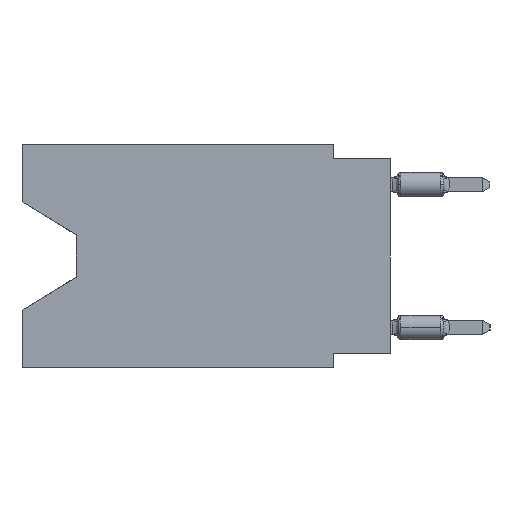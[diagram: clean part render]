
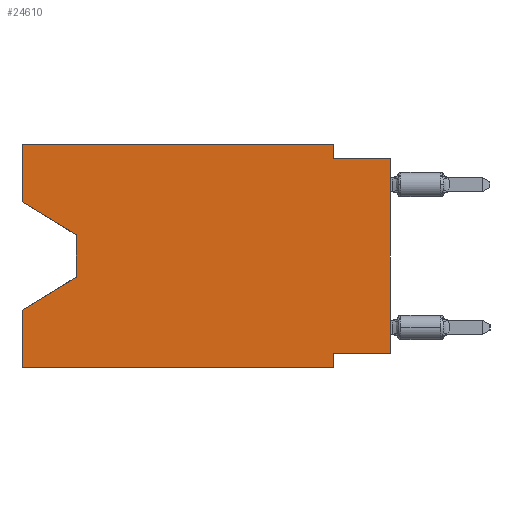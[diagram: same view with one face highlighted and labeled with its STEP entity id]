
A CAD part, left-side view. The second image highlights one B-rep face of the part: STEP entity #24610.
In plain terms, the highlighted planar face has unit normal (-1, 0, 0).
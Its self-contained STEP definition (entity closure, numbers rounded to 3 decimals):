
#326 = CARTESIAN_POINT ( 'NONE',  ( 0., 0., 0. ) ) ;
#1478 = CARTESIAN_POINT ( 'NONE',  ( 0., 16.383, -9.906 ) ) ;
#2300 = EDGE_CURVE ( 'NONE', #13877, #27841, #21555, .T. ) ;
#2341 = ORIENTED_EDGE ( 'NONE', *, *, #12382, .T. ) ;
#2949 = DIRECTION ( 'NONE',  ( 0., -1., 0. ) ) ;
#4019 = CARTESIAN_POINT ( 'NONE',  ( 0., 16.383, 0. ) ) ;
#5194 = VECTOR ( 'NONE', #12297, 1000. ) ;
#5306 = LINE ( 'NONE', #8620, #13654 ) ;
#5912 = VERTEX_POINT ( 'NONE', #15106 ) ;
#6220 = VECTOR ( 'NONE', #15846, 1000. ) ;
#6230 = EDGE_CURVE ( 'NONE', #9667, #5912, #23600, .T. ) ;
#7254 = AXIS2_PLACEMENT_3D ( 'NONE', #31137, #18847, #9213 ) ;
#7449 = CARTESIAN_POINT ( 'NONE',  ( 0., 0., -0.635 ) ) ;
#7759 = DIRECTION ( 'NONE',  ( 0., 0., 1. ) ) ;
#7861 = CARTESIAN_POINT ( 'NONE',  ( 0., 2.54, -9.271 ) ) ;
#7960 = VERTEX_POINT ( 'NONE', #19736 ) ;
#8156 = DIRECTION ( 'NONE',  ( 0., 0., 1. ) ) ;
#8190 = LINE ( 'NONE', #27439, #19016 ) ;
#8208 = ORIENTED_EDGE ( 'NONE', *, *, #6230, .F. ) ;
#8586 = VECTOR ( 'NONE', #8156, 1000. ) ;
#8620 = CARTESIAN_POINT ( 'NONE',  ( 0., 13.97, -5.893 ) ) ;
#8737 = CARTESIAN_POINT ( 'NONE',  ( 0., 16.383, -2.546 ) ) ;
#9008 = VECTOR ( 'NONE', #30853, 1000. ) ;
#9213 = DIRECTION ( 'NONE',  ( 0., 0., -1. ) ) ;
#9254 = DIRECTION ( 'NONE',  ( 0., 0., -1. ) ) ;
#9667 = VERTEX_POINT ( 'NONE', #7861 ) ;
#9680 = PLANE ( 'NONE',  #7254 ) ;
#10047 = LINE ( 'NONE', #1478, #26057 ) ;
#10245 = VECTOR ( 'NONE', #9254, 1000. ) ;
#10499 = DIRECTION ( 'NONE',  ( 0., 0.855, -0.519 ) ) ;
#11069 = VERTEX_POINT ( 'NONE', #30880 ) ;
#11603 = CARTESIAN_POINT ( 'NONE',  ( 0., 2.54, -9.906 ) ) ;
#12297 = DIRECTION ( 'NONE',  ( 0., -0.855, -0.519 ) ) ;
#12382 = EDGE_CURVE ( 'NONE', #27841, #31205, #5306, .T. ) ;
#12437 = ORIENTED_EDGE ( 'NONE', *, *, #2300, .T. ) ;
#12693 = CARTESIAN_POINT ( 'NONE',  ( 0., 13.97, -4.013 ) ) ;
#13144 = EDGE_CURVE ( 'NONE', #11069, #30994, #14709, .T. ) ;
#13451 = CARTESIAN_POINT ( 'NONE',  ( 0., 16.383, -7.36 ) ) ;
#13635 = ORIENTED_EDGE ( 'NONE', *, *, #25833, .F. ) ;
#13641 = EDGE_CURVE ( 'NONE', #26118, #16087, #27875, .T. ) ;
#13654 = VECTOR ( 'NONE', #10499, 1000. ) ;
#13877 = VERTEX_POINT ( 'NONE', #12693 ) ;
#14334 = VECTOR ( 'NONE', #23282, 1000. ) ;
#14366 = LINE ( 'NONE', #28882, #5194 ) ;
#14709 = LINE ( 'NONE', #326, #20678 ) ;
#15106 = CARTESIAN_POINT ( 'NONE',  ( 0., 2.54, -9.906 ) ) ;
#15130 = EDGE_CURVE ( 'NONE', #31153, #5912, #10047, .T. ) ;
#15409 = CARTESIAN_POINT ( 'NONE',  ( 0., 16.383, 0. ) ) ;
#15824 = CARTESIAN_POINT ( 'NONE',  ( 0., 16.383, -9.906 ) ) ;
#15846 = DIRECTION ( 'NONE',  ( 0., 0., 1. ) ) ;
#16087 = VERTEX_POINT ( 'NONE', #30303 ) ;
#17230 = LINE ( 'NONE', #7449, #30895 ) ;
#18193 = CARTESIAN_POINT ( 'NONE',  ( 0., 13.97, -5.893 ) ) ;
#18832 = LINE ( 'NONE', #28458, #6220 ) ;
#18847 = DIRECTION ( 'NONE',  ( 1., 0., 0. ) ) ;
#19016 = VECTOR ( 'NONE', #25064, 1000. ) ;
#19604 = ORIENTED_EDGE ( 'NONE', *, *, #15130, .T. ) ;
#19736 = CARTESIAN_POINT ( 'NONE',  ( 0., 2.54, -0.635 ) ) ;
#20631 = CARTESIAN_POINT ( 'NONE',  ( 0., 2.54, 0. ) ) ;
#20678 = VECTOR ( 'NONE', #7759, 1000. ) ;
#20753 = EDGE_CURVE ( 'NONE', #31153, #31205, #18832, .T. ) ;
#20844 = EDGE_CURVE ( 'NONE', #7960, #30994, #17230, .T. ) ;
#21297 = EDGE_CURVE ( 'NONE', #26118, #13877, #14366, .T. ) ;
#21345 = ORIENTED_EDGE ( 'NONE', *, *, #13144, .T. ) ;
#21555 = LINE ( 'NONE', #28512, #10245 ) ;
#21976 = CARTESIAN_POINT ( 'NONE',  ( 0., 0., -0.635 ) ) ;
#22077 = ORIENTED_EDGE ( 'NONE', *, *, #20844, .F. ) ;
#23282 = DIRECTION ( 'NONE',  ( 0., -1., 0. ) ) ;
#23460 = ORIENTED_EDGE ( 'NONE', *, *, #20753, .F. ) ;
#23600 = LINE ( 'NONE', #11603, #9008 ) ;
#23917 = ORIENTED_EDGE ( 'NONE', *, *, #29962, .F. ) ;
#24467 = EDGE_CURVE ( 'NONE', #16087, #27168, #25177, .T. ) ;
#24502 = DIRECTION ( 'NONE',  ( 0., -1., 0. ) ) ;
#24573 = ORIENTED_EDGE ( 'NONE', *, *, #24467, .F. ) ;
#24610 = ADVANCED_FACE ( 'NONE', ( #28326 ), #9680, .F. ) ;
#25046 = EDGE_LOOP ( 'NONE', ( #25277, #12437, #2341, #23460, #19604, #8208, #13635, #21345, #22077, #23917, #24573, #27408 ) ) ;
#25064 = DIRECTION ( 'NONE',  ( 0., 0., -1. ) ) ;
#25177 = LINE ( 'NONE', #4019, #14334 ) ;
#25277 = ORIENTED_EDGE ( 'NONE', *, *, #21297, .T. ) ;
#25833 = EDGE_CURVE ( 'NONE', #11069, #9667, #26417, .T. ) ;
#26057 = VECTOR ( 'NONE', #2949, 1000. ) ;
#26118 = VERTEX_POINT ( 'NONE', #8737 ) ;
#26417 = LINE ( 'NONE', #26563, #29997 ) ;
#26563 = CARTESIAN_POINT ( 'NONE',  ( 0., 0., -9.271 ) ) ;
#27168 = VERTEX_POINT ( 'NONE', #20631 ) ;
#27408 = ORIENTED_EDGE ( 'NONE', *, *, #13641, .F. ) ;
#27439 = CARTESIAN_POINT ( 'NONE',  ( 0., 2.54, 0. ) ) ;
#27841 = VERTEX_POINT ( 'NONE', #18193 ) ;
#27875 = LINE ( 'NONE', #15409, #8586 ) ;
#28326 = FACE_OUTER_BOUND ( 'NONE', #25046, .T. ) ;
#28458 = CARTESIAN_POINT ( 'NONE',  ( 0., 16.383, 0. ) ) ;
#28512 = CARTESIAN_POINT ( 'NONE',  ( 0., 13.97, -4.013 ) ) ;
#28882 = CARTESIAN_POINT ( 'NONE',  ( 0., 16.383, -2.546 ) ) ;
#29962 = EDGE_CURVE ( 'NONE', #27168, #7960, #8190, .T. ) ;
#29997 = VECTOR ( 'NONE', #31143, 1000. ) ;
#30303 = CARTESIAN_POINT ( 'NONE',  ( 0., 16.383, 0. ) ) ;
#30853 = DIRECTION ( 'NONE',  ( 0., 0., -1. ) ) ;
#30880 = CARTESIAN_POINT ( 'NONE',  ( 0., 0., -9.271 ) ) ;
#30895 = VECTOR ( 'NONE', #24502, 1000. ) ;
#30994 = VERTEX_POINT ( 'NONE', #21976 ) ;
#31137 = CARTESIAN_POINT ( 'NONE',  ( 0., 16.383, 0. ) ) ;
#31143 = DIRECTION ( 'NONE',  ( 0., 1., 0. ) ) ;
#31153 = VERTEX_POINT ( 'NONE', #15824 ) ;
#31205 = VERTEX_POINT ( 'NONE', #13451 ) ;
